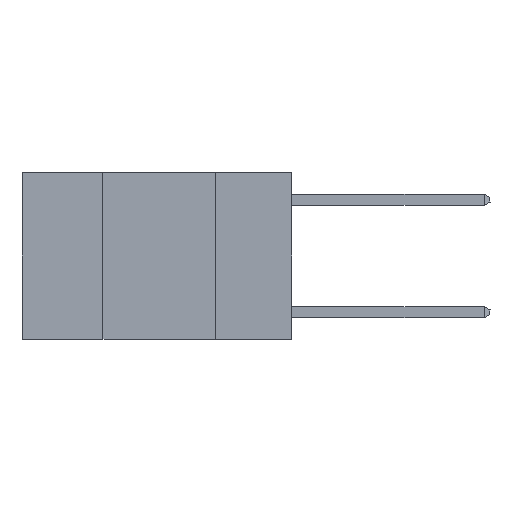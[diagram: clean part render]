
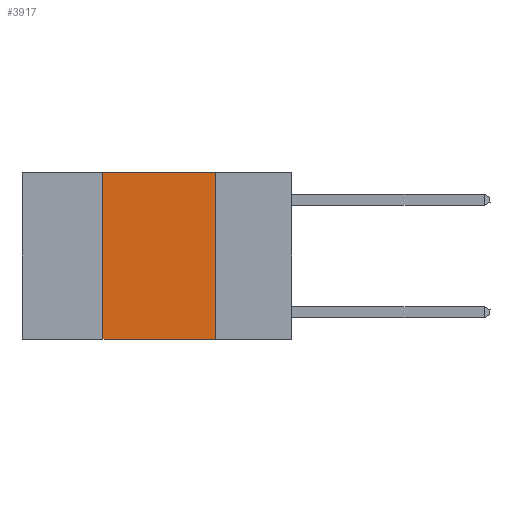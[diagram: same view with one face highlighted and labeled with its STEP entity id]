
A CAD part, left-side view. The second image highlights one B-rep face of the part: STEP entity #3917.
In plain terms, the highlighted planar face has unit normal (-1, 0, 0).
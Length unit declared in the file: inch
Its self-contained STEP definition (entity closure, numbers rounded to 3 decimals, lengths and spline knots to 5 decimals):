
#13 = EDGE_CURVE ( 'NONE', #9226, #4642, #663, .T. ) ;
#20 = VERTEX_POINT ( 'NONE', #8855 ) ;
#143 = ORIENTED_EDGE ( 'NONE', *, *, #8420, .F. ) ;
#254 = PLANE ( 'NONE',  #11356 ) ;
#332 = ORIENTED_EDGE ( 'NONE', *, *, #13, .F. ) ;
#416 = LINE ( 'NONE', #8535, #2483 ) ;
#624 = VECTOR ( 'NONE', #4410, 39.37008 ) ;
#663 = LINE ( 'NONE', #3576, #624 ) ;
#2379 = DIRECTION ( 'NONE',  ( 0., 0., -1. ) ) ;
#2483 = VECTOR ( 'NONE', #3923, 39.37008 ) ;
#2610 = DIRECTION ( 'NONE',  ( 0., -1., 0. ) ) ;
#2816 = VECTOR ( 'NONE', #2379, 39.37008 ) ;
#3168 = EDGE_LOOP ( 'NONE', ( #143, #4119, #332, #4728 ) ) ;
#3474 = CARTESIAN_POINT ( 'NONE',  ( 0., 0.42, -0.37 ) ) ;
#3576 = CARTESIAN_POINT ( 'NONE',  ( 0., 0.42, 0. ) ) ;
#3917 = ADVANCED_FACE ( 'NONE', ( #6740 ), #254, .F. ) ;
#3923 = DIRECTION ( 'NONE',  ( 0., -1., 0. ) ) ;
#4119 = ORIENTED_EDGE ( 'NONE', *, *, #10127, .F. ) ;
#4127 = VERTEX_POINT ( 'NONE', #6847 ) ;
#4410 = DIRECTION ( 'NONE',  ( 0., 0., 1. ) ) ;
#4642 = VERTEX_POINT ( 'NONE', #7071 ) ;
#4728 = ORIENTED_EDGE ( 'NONE', *, *, #10476, .T. ) ;
#5375 = CARTESIAN_POINT ( 'NONE',  ( 0., 0.6, 0. ) ) ;
#5425 = DIRECTION ( 'NONE',  ( 0., 0., -1. ) ) ;
#6010 = VECTOR ( 'NONE', #2610, 39.37008 ) ;
#6740 = FACE_OUTER_BOUND ( 'NONE', #3168, .T. ) ;
#6847 = CARTESIAN_POINT ( 'NONE',  ( 0., 0.17, 0. ) ) ;
#7071 = CARTESIAN_POINT ( 'NONE',  ( 0., 0.42, 0. ) ) ;
#7484 = LINE ( 'NONE', #7938, #2816 ) ;
#7938 = CARTESIAN_POINT ( 'NONE',  ( 0., 0.17, 0. ) ) ;
#8420 = EDGE_CURVE ( 'NONE', #4127, #20, #7484, .T. ) ;
#8535 = CARTESIAN_POINT ( 'NONE',  ( 0., 0.6, -0.37 ) ) ;
#8855 = CARTESIAN_POINT ( 'NONE',  ( 0., 0.17, -0.37 ) ) ;
#9226 = VERTEX_POINT ( 'NONE', #3474 ) ;
#10127 = EDGE_CURVE ( 'NONE', #4642, #4127, #10644, .T. ) ;
#10318 = DIRECTION ( 'NONE',  ( 1., 0., 0. ) ) ;
#10476 = EDGE_CURVE ( 'NONE', #9226, #20, #416, .T. ) ;
#10644 = LINE ( 'NONE', #10696, #6010 ) ;
#10696 = CARTESIAN_POINT ( 'NONE',  ( 0., 0.6, 0. ) ) ;
#11356 = AXIS2_PLACEMENT_3D ( 'NONE', #5375, #10318, #5425 ) ;
